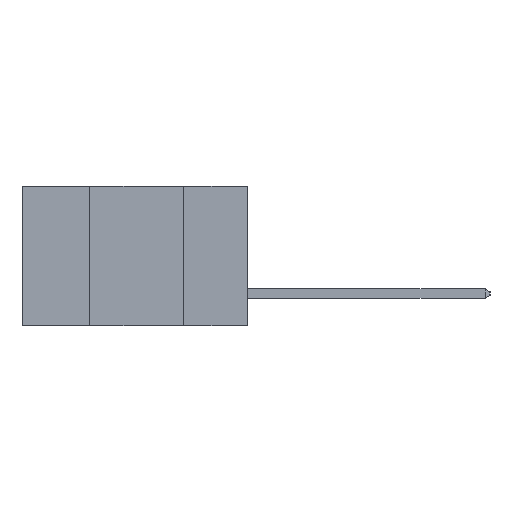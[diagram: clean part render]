
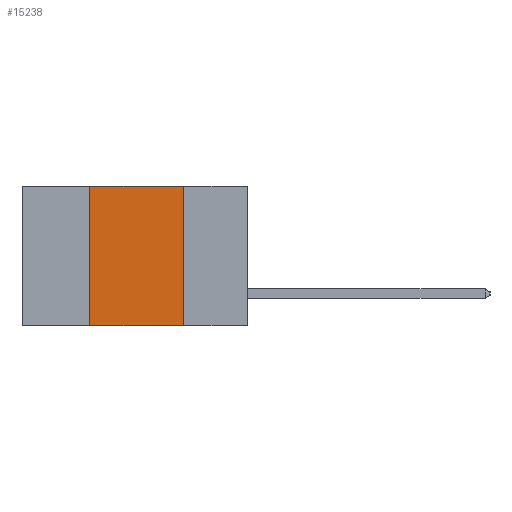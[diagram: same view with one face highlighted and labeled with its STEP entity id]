
A CAD part, left-side view. The second image highlights one B-rep face of the part: STEP entity #15238.
In plain terms, the highlighted planar face has unit normal (-1, 0, 0).
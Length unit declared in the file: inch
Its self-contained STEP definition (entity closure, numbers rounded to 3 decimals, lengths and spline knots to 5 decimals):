
#50 = EDGE_CURVE ( 'NONE', #1352, #10550, #12887, .T. ) ;
#117 = ORIENTED_EDGE ( 'NONE', *, *, #4765, .F. ) ;
#1352 = VERTEX_POINT ( 'NONE', #5301 ) ;
#1424 = ORIENTED_EDGE ( 'NONE', *, *, #50, .T. ) ;
#1436 = DIRECTION ( 'NONE',  ( 0., 0., 1. ) ) ;
#1941 = EDGE_CURVE ( 'NONE', #1352, #9153, #6746, .T. ) ;
#1954 = CARTESIAN_POINT ( 'NONE',  ( 0., 0.17, 0. ) ) ;
#2342 = DIRECTION ( 'NONE',  ( 0., 0., -1. ) ) ;
#2921 = VECTOR ( 'NONE', #1436, 39.37008 ) ;
#3229 = VERTEX_POINT ( 'NONE', #1954 ) ;
#3442 = EDGE_LOOP ( 'NONE', ( #117, #4323, #4741, #1424 ) ) ;
#4003 = DIRECTION ( 'NONE',  ( 0., 0., -1. ) ) ;
#4323 = ORIENTED_EDGE ( 'NONE', *, *, #4690, .F. ) ;
#4690 = EDGE_CURVE ( 'NONE', #9153, #3229, #11409, .T. ) ;
#4741 = ORIENTED_EDGE ( 'NONE', *, *, #1941, .F. ) ;
#4765 = EDGE_CURVE ( 'NONE', #3229, #10550, #13621, .T. ) ;
#5301 = CARTESIAN_POINT ( 'NONE',  ( 0., 0.42, -0.37 ) ) ;
#6157 = FACE_OUTER_BOUND ( 'NONE', #3442, .T. ) ;
#6746 = LINE ( 'NONE', #8340, #2921 ) ;
#7466 = CARTESIAN_POINT ( 'NONE',  ( 0., 0.17, 0. ) ) ;
#7912 = VECTOR ( 'NONE', #9602, 39.37008 ) ;
#8218 = CARTESIAN_POINT ( 'NONE',  ( 0., 0.6, -0.37 ) ) ;
#8340 = CARTESIAN_POINT ( 'NONE',  ( 0., 0.42, 0. ) ) ;
#9153 = VERTEX_POINT ( 'NONE', #10917 ) ;
#9410 = VECTOR ( 'NONE', #13142, 39.37008 ) ;
#9602 = DIRECTION ( 'NONE',  ( 0., -1., 0. ) ) ;
#10550 = VERTEX_POINT ( 'NONE', #13865 ) ;
#10653 = PLANE ( 'NONE',  #12017 ) ;
#10770 = CARTESIAN_POINT ( 'NONE',  ( 0., 0.6, 0. ) ) ;
#10917 = CARTESIAN_POINT ( 'NONE',  ( 0., 0.42, 0. ) ) ;
#11409 = LINE ( 'NONE', #10770, #7912 ) ;
#11973 = DIRECTION ( 'NONE',  ( 1., 0., 0. ) ) ;
#12017 = AXIS2_PLACEMENT_3D ( 'NONE', #15768, #11973, #4003 ) ;
#12887 = LINE ( 'NONE', #8218, #9410 ) ;
#13142 = DIRECTION ( 'NONE',  ( 0., -1., 0. ) ) ;
#13621 = LINE ( 'NONE', #7466, #16611 ) ;
#13865 = CARTESIAN_POINT ( 'NONE',  ( 0., 0.17, -0.37 ) ) ;
#15238 = ADVANCED_FACE ( 'NONE', ( #6157 ), #10653, .F. ) ;
#15768 = CARTESIAN_POINT ( 'NONE',  ( 0., 0.6, 0. ) ) ;
#16611 = VECTOR ( 'NONE', #2342, 39.37008 ) ;
